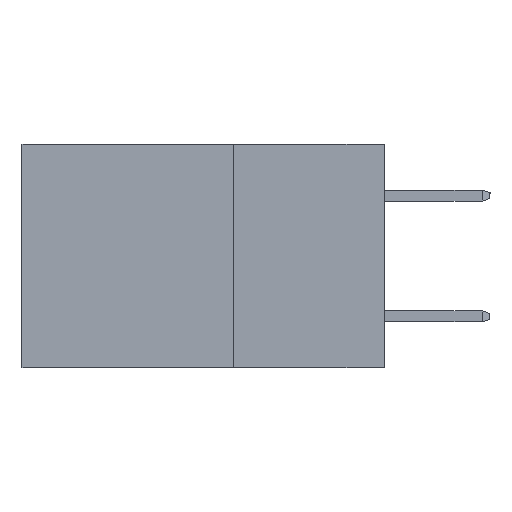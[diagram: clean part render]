
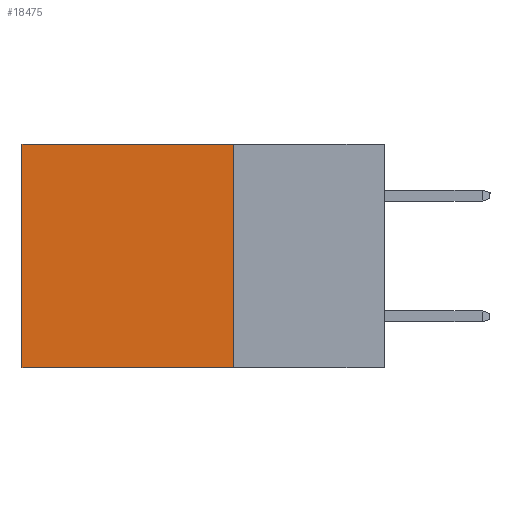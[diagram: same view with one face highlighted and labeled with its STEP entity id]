
A CAD part, left-side view. The second image highlights one B-rep face of the part: STEP entity #18475.
In plain terms, the highlighted planar face has unit normal (-1, 0, 0).
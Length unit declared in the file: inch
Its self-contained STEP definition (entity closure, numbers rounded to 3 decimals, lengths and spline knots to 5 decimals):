
#672 = ORIENTED_EDGE ( 'NONE', *, *, #13268, .F. ) ;
#888 = VERTEX_POINT ( 'NONE', #6448 ) ;
#1075 = CARTESIAN_POINT ( 'NONE',  ( 0.2615, 0.25, -0.37 ) ) ;
#1702 = DIRECTION ( 'NONE',  ( 0., 1., 0. ) ) ;
#2112 = LINE ( 'NONE', #2433, #12227 ) ;
#2222 = VERTEX_POINT ( 'NONE', #18789 ) ;
#2255 = CARTESIAN_POINT ( 'NONE',  ( 0.2615, 0.6, 0. ) ) ;
#2433 = CARTESIAN_POINT ( 'NONE',  ( 0.2615, 0.25, -0.37 ) ) ;
#2946 = DIRECTION ( 'NONE',  ( 0., 0., -1. ) ) ;
#3918 = EDGE_CURVE ( 'NONE', #888, #11137, #16022, .T. ) ;
#4151 = EDGE_LOOP ( 'NONE', ( #20458, #672, #18219, #12645 ) ) ;
#5378 = LINE ( 'NONE', #8744, #9200 ) ;
#6448 = CARTESIAN_POINT ( 'NONE',  ( 0.2615, 0.25, 0. ) ) ;
#7591 = DIRECTION ( 'NONE',  ( 0., 0., -1. ) ) ;
#8130 = CARTESIAN_POINT ( 'NONE',  ( 0.2615, 0.25, -0.37 ) ) ;
#8277 = VERTEX_POINT ( 'NONE', #1075 ) ;
#8744 = CARTESIAN_POINT ( 'NONE',  ( 0.2615, 0.25, -0.37 ) ) ;
#9200 = VECTOR ( 'NONE', #1702, 39.37008 ) ;
#11137 = VERTEX_POINT ( 'NONE', #2255 ) ;
#11312 = CARTESIAN_POINT ( 'NONE',  ( 0.2615, 0.6, -0.37 ) ) ;
#11422 = DIRECTION ( 'NONE',  ( 0., 0., -1. ) ) ;
#11724 = VECTOR ( 'NONE', #14091, 39.37008 ) ;
#12227 = VECTOR ( 'NONE', #7591, 39.37008 ) ;
#12645 = ORIENTED_EDGE ( 'NONE', *, *, #3918, .T. ) ;
#13045 = FACE_OUTER_BOUND ( 'NONE', #4151, .T. ) ;
#13104 = LINE ( 'NONE', #11312, #18362 ) ;
#13268 = EDGE_CURVE ( 'NONE', #8277, #2222, #5378, .T. ) ;
#14091 = DIRECTION ( 'NONE',  ( 0., 1., 0. ) ) ;
#15203 = EDGE_CURVE ( 'NONE', #888, #8277, #2112, .T. ) ;
#16022 = LINE ( 'NONE', #19587, #11724 ) ;
#16636 = DIRECTION ( 'NONE',  ( 1., 0., 0. ) ) ;
#18219 = ORIENTED_EDGE ( 'NONE', *, *, #15203, .F. ) ;
#18362 = VECTOR ( 'NONE', #11422, 39.37008 ) ;
#18475 = ADVANCED_FACE ( 'NONE', ( #13045 ), #22031, .F. ) ;
#18789 = CARTESIAN_POINT ( 'NONE',  ( 0.2615, 0.6, -0.37 ) ) ;
#18860 = EDGE_CURVE ( 'NONE', #11137, #2222, #13104, .T. ) ;
#19587 = CARTESIAN_POINT ( 'NONE',  ( 0.2615, 0.25, 0. ) ) ;
#20458 = ORIENTED_EDGE ( 'NONE', *, *, #18860, .T. ) ;
#21594 = AXIS2_PLACEMENT_3D ( 'NONE', #8130, #16636, #2946 ) ;
#22031 = PLANE ( 'NONE',  #21594 ) ;
